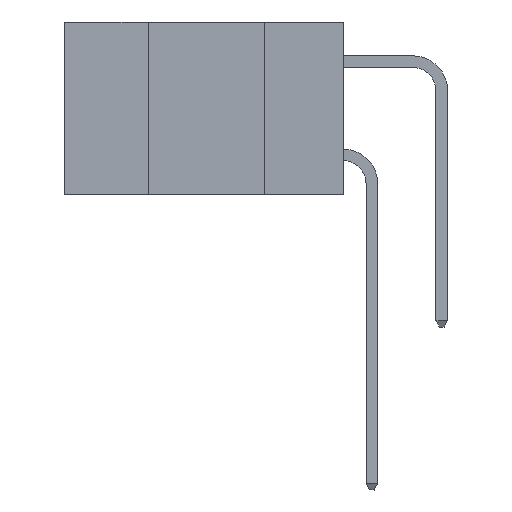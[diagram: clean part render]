
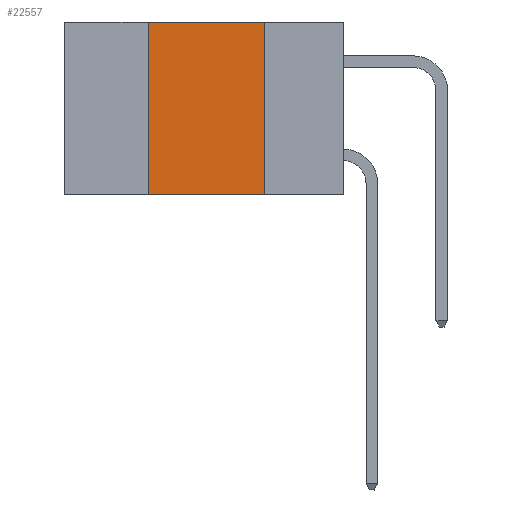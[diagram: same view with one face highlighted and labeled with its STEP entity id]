
A CAD part, left-side view. The second image highlights one B-rep face of the part: STEP entity #22557.
In plain terms, the highlighted planar face has unit normal (-1, 0, 0).
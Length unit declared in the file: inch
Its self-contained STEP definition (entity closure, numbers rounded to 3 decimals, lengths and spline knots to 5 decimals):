
#1390 = CARTESIAN_POINT ( 'NONE',  ( 0., 0.42, -0.37 ) ) ;
#1647 = VERTEX_POINT ( 'NONE', #13311 ) ;
#2078 = VERTEX_POINT ( 'NONE', #24943 ) ;
#2745 = CARTESIAN_POINT ( 'NONE',  ( 0., 0.17, 0. ) ) ;
#2974 = EDGE_CURVE ( 'NONE', #7159, #1647, #12345, .T. ) ;
#3343 = DIRECTION ( 'NONE',  ( 1., 0., 0. ) ) ;
#3474 = PLANE ( 'NONE',  #5948 ) ;
#4606 = ORIENTED_EDGE ( 'NONE', *, *, #9771, .F. ) ;
#5194 = LINE ( 'NONE', #1390, #22797 ) ;
#5948 = AXIS2_PLACEMENT_3D ( 'NONE', #22003, #3343, #11664 ) ;
#7159 = VERTEX_POINT ( 'NONE', #17011 ) ;
#8255 = ORIENTED_EDGE ( 'NONE', *, *, #21358, .F. ) ;
#9642 = VERTEX_POINT ( 'NONE', #2745 ) ;
#9771 = EDGE_CURVE ( 'NONE', #7159, #2078, #5194, .T. ) ;
#9791 = VECTOR ( 'NONE', #20536, 39.37008 ) ;
#10301 = LINE ( 'NONE', #22815, #21560 ) ;
#10592 = CARTESIAN_POINT ( 'NONE',  ( 0., 0.6, 0. ) ) ;
#10882 = VECTOR ( 'NONE', #14512, 39.37008 ) ;
#11664 = DIRECTION ( 'NONE',  ( 0., 0., -1. ) ) ;
#11681 = ORIENTED_EDGE ( 'NONE', *, *, #18439, .F. ) ;
#12241 = LINE ( 'NONE', #10592, #9791 ) ;
#12345 = LINE ( 'NONE', #12607, #10882 ) ;
#12607 = CARTESIAN_POINT ( 'NONE',  ( 0., 0.6, -0.37 ) ) ;
#13311 = CARTESIAN_POINT ( 'NONE',  ( 0., 0.17, -0.37 ) ) ;
#14512 = DIRECTION ( 'NONE',  ( 0., -1., 0. ) ) ;
#14887 = DIRECTION ( 'NONE',  ( 0., 0., -1. ) ) ;
#16001 = FACE_OUTER_BOUND ( 'NONE', #26590, .T. ) ;
#17011 = CARTESIAN_POINT ( 'NONE',  ( 0., 0.42, -0.37 ) ) ;
#18439 = EDGE_CURVE ( 'NONE', #2078, #9642, #12241, .T. ) ;
#20536 = DIRECTION ( 'NONE',  ( 0., -1., 0. ) ) ;
#21358 = EDGE_CURVE ( 'NONE', #9642, #1647, #10301, .T. ) ;
#21560 = VECTOR ( 'NONE', #14887, 39.37008 ) ;
#21823 = DIRECTION ( 'NONE',  ( 0., 0., 1. ) ) ;
#22003 = CARTESIAN_POINT ( 'NONE',  ( 0., 0.6, 0. ) ) ;
#22557 = ADVANCED_FACE ( 'NONE', ( #16001 ), #3474, .F. ) ;
#22797 = VECTOR ( 'NONE', #21823, 39.37008 ) ;
#22815 = CARTESIAN_POINT ( 'NONE',  ( 0., 0.17, -0.37 ) ) ;
#24943 = CARTESIAN_POINT ( 'NONE',  ( 0., 0.42, 0. ) ) ;
#26307 = ORIENTED_EDGE ( 'NONE', *, *, #2974, .T. ) ;
#26590 = EDGE_LOOP ( 'NONE', ( #8255, #11681, #4606, #26307 ) ) ;
